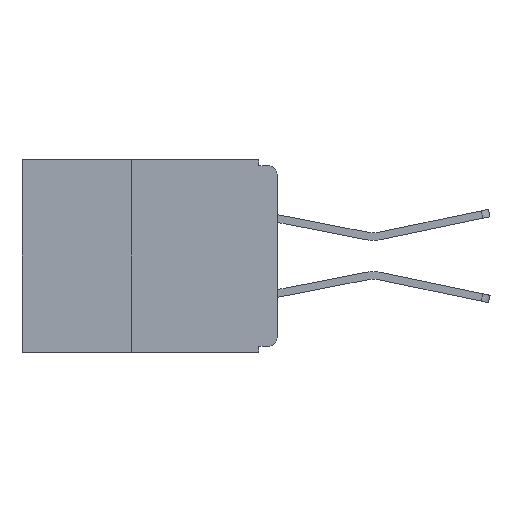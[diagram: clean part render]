
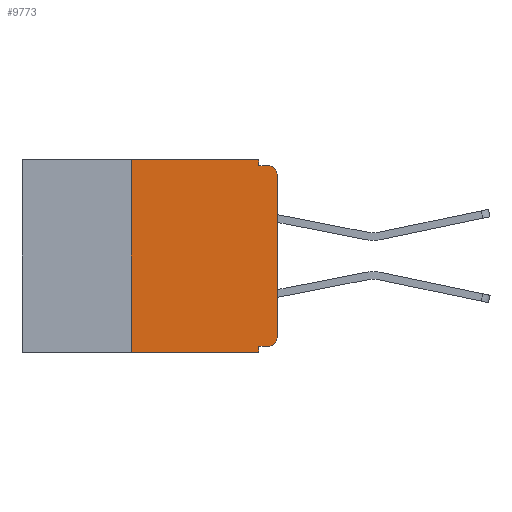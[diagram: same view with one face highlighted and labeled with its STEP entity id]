
A CAD part, left-side view. The second image highlights one B-rep face of the part: STEP entity #9773.
In plain terms, the highlighted planar face has unit normal (-1, 0, 0).
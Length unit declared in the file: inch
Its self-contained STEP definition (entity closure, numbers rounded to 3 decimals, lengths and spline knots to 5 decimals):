
#388 = EDGE_CURVE ( 'NONE', #6679, #8734, #11144, .T. ) ;
#430 = ORIENTED_EDGE ( 'NONE', *, *, #2406, .F. ) ;
#595 = CARTESIAN_POINT ( 'NONE',  ( 0., 0.25, -0.33 ) ) ;
#730 = LINE ( 'NONE', #12805, #9682 ) ;
#848 = CARTESIAN_POINT ( 'NONE',  ( 0., 0., 0. ) ) ;
#1160 = CARTESIAN_POINT ( 'NONE',  ( 0., 0., -0.025 ) ) ;
#1294 = VERTEX_POINT ( 'NONE', #9336 ) ;
#1824 = PLANE ( 'NONE',  #2856 ) ;
#1891 = CARTESIAN_POINT ( 'NONE',  ( 0., 0., -0.32 ) ) ;
#1994 = CARTESIAN_POINT ( 'NONE',  ( 0., 0.031, 0. ) ) ;
#2049 = CARTESIAN_POINT ( 'NONE',  ( 0., 0.031, -0.32 ) ) ;
#2096 = DIRECTION ( 'NONE',  ( 0., 0., 1. ) ) ;
#2225 = DIRECTION ( 'NONE',  ( -1., 0., 0. ) ) ;
#2396 = CARTESIAN_POINT ( 'NONE',  ( 0., 0.031, 0. ) ) ;
#2406 = EDGE_CURVE ( 'NONE', #8734, #5969, #11258, .T. ) ;
#2742 = ORIENTED_EDGE ( 'NONE', *, *, #388, .F. ) ;
#2856 = AXIS2_PLACEMENT_3D ( 'NONE', #3118, #4327, #12711 ) ;
#2888 = DIRECTION ( 'NONE',  ( -1., 0., 0. ) ) ;
#2902 = VERTEX_POINT ( 'NONE', #2396 ) ;
#3002 = DIRECTION ( 'NONE',  ( 0., -1., 0. ) ) ;
#3118 = CARTESIAN_POINT ( 'NONE',  ( 0., 0.437, 0. ) ) ;
#3169 = VECTOR ( 'NONE', #10469, 39.37008 ) ;
#3208 = DIRECTION ( 'NONE',  ( 0., -1., 0. ) ) ;
#3241 = ORIENTED_EDGE ( 'NONE', *, *, #5230, .F. ) ;
#3298 = CARTESIAN_POINT ( 'NONE',  ( 0., 0.25, -0.33 ) ) ;
#3514 = VERTEX_POINT ( 'NONE', #13045 ) ;
#3628 = ORIENTED_EDGE ( 'NONE', *, *, #15237, .T. ) ;
#3642 = CARTESIAN_POINT ( 'NONE',  ( 0., 0.015, -0.01 ) ) ;
#4010 = CIRCLE ( 'NONE', #7368, 0.015 ) ;
#4327 = DIRECTION ( 'NONE',  ( 1., 0., 0. ) ) ;
#4336 = VERTEX_POINT ( 'NONE', #9808 ) ;
#4572 = CARTESIAN_POINT ( 'NONE',  ( 0., 0.031, -0.33 ) ) ;
#4638 = ORIENTED_EDGE ( 'NONE', *, *, #5960, .T. ) ;
#5230 = EDGE_CURVE ( 'NONE', #1294, #2902, #730, .T. ) ;
#5712 = EDGE_CURVE ( 'NONE', #6679, #4336, #4010, .T. ) ;
#5951 = VERTEX_POINT ( 'NONE', #3298 ) ;
#5960 = EDGE_CURVE ( 'NONE', #4336, #12733, #12627, .T. ) ;
#5969 = VERTEX_POINT ( 'NONE', #4572 ) ;
#6125 = LINE ( 'NONE', #13078, #11760 ) ;
#6263 = AXIS2_PLACEMENT_3D ( 'NONE', #9485, #2225, #10691 ) ;
#6606 = CARTESIAN_POINT ( 'NONE',  ( 0., 0., -0.01 ) ) ;
#6679 = VERTEX_POINT ( 'NONE', #9556 ) ;
#7100 = DIRECTION ( 'NONE',  ( 0., -1., 0. ) ) ;
#7368 = AXIS2_PLACEMENT_3D ( 'NONE', #10113, #2888, #11316 ) ;
#7591 = EDGE_CURVE ( 'NONE', #5951, #1294, #9066, .T. ) ;
#7763 = ORIENTED_EDGE ( 'NONE', *, *, #8685, .F. ) ;
#7861 = CIRCLE ( 'NONE', #6263, 0.015 ) ;
#8685 = EDGE_CURVE ( 'NONE', #2902, #3514, #9207, .T. ) ;
#8734 = VERTEX_POINT ( 'NONE', #2049 ) ;
#8958 = VECTOR ( 'NONE', #3002, 39.37008 ) ;
#9044 = ORIENTED_EDGE ( 'NONE', *, *, #5712, .T. ) ;
#9066 = LINE ( 'NONE', #595, #14946 ) ;
#9111 = DIRECTION ( 'NONE',  ( 0., 0., 1. ) ) ;
#9207 = LINE ( 'NONE', #1994, #3169 ) ;
#9336 = CARTESIAN_POINT ( 'NONE',  ( 0., 0.25, 0. ) ) ;
#9485 = CARTESIAN_POINT ( 'NONE',  ( 0., 0.015, -0.025 ) ) ;
#9491 = EDGE_LOOP ( 'NONE', ( #4638, #3628, #13897, #7763, #3241, #13611, #11483, #430, #2742, #9044 ) ) ;
#9556 = CARTESIAN_POINT ( 'NONE',  ( 0., 0.015, -0.32 ) ) ;
#9682 = VECTOR ( 'NONE', #3208, 39.37008 ) ;
#9773 = ADVANCED_FACE ( 'NONE', ( #13966 ), #1824, .F. ) ;
#9808 = CARTESIAN_POINT ( 'NONE',  ( 0., 0., -0.305 ) ) ;
#9839 = VECTOR ( 'NONE', #2096, 39.37008 ) ;
#10113 = CARTESIAN_POINT ( 'NONE',  ( 0., 0.015, -0.305 ) ) ;
#10367 = EDGE_CURVE ( 'NONE', #3514, #11520, #12149, .T. ) ;
#10469 = DIRECTION ( 'NONE',  ( 0., 0., -1. ) ) ;
#10691 = DIRECTION ( 'NONE',  ( 0., 0., -1. ) ) ;
#10813 = EDGE_CURVE ( 'NONE', #5951, #5969, #6125, .T. ) ;
#11144 = LINE ( 'NONE', #1891, #14591 ) ;
#11258 = LINE ( 'NONE', #13476, #14000 ) ;
#11316 = DIRECTION ( 'NONE',  ( 0., 0., -1. ) ) ;
#11483 = ORIENTED_EDGE ( 'NONE', *, *, #10813, .T. ) ;
#11520 = VERTEX_POINT ( 'NONE', #3642 ) ;
#11760 = VECTOR ( 'NONE', #7100, 39.37008 ) ;
#12149 = LINE ( 'NONE', #6606, #8958 ) ;
#12627 = LINE ( 'NONE', #848, #9839 ) ;
#12711 = DIRECTION ( 'NONE',  ( 0., 0., -1. ) ) ;
#12733 = VERTEX_POINT ( 'NONE', #1160 ) ;
#12805 = CARTESIAN_POINT ( 'NONE',  ( 0., 0.437, 0. ) ) ;
#13045 = CARTESIAN_POINT ( 'NONE',  ( 0., 0.031, -0.01 ) ) ;
#13078 = CARTESIAN_POINT ( 'NONE',  ( 0., 0.437, -0.33 ) ) ;
#13476 = CARTESIAN_POINT ( 'NONE',  ( 0., 0.031, -0.33 ) ) ;
#13532 = DIRECTION ( 'NONE',  ( 0., 0., -1. ) ) ;
#13611 = ORIENTED_EDGE ( 'NONE', *, *, #7591, .F. ) ;
#13897 = ORIENTED_EDGE ( 'NONE', *, *, #10367, .F. ) ;
#13966 = FACE_OUTER_BOUND ( 'NONE', #9491, .T. ) ;
#14000 = VECTOR ( 'NONE', #13532, 39.37008 ) ;
#14591 = VECTOR ( 'NONE', #14769, 39.37008 ) ;
#14769 = DIRECTION ( 'NONE',  ( 0., 1., 0. ) ) ;
#14946 = VECTOR ( 'NONE', #9111, 39.37008 ) ;
#15237 = EDGE_CURVE ( 'NONE', #12733, #11520, #7861, .T. ) ;
